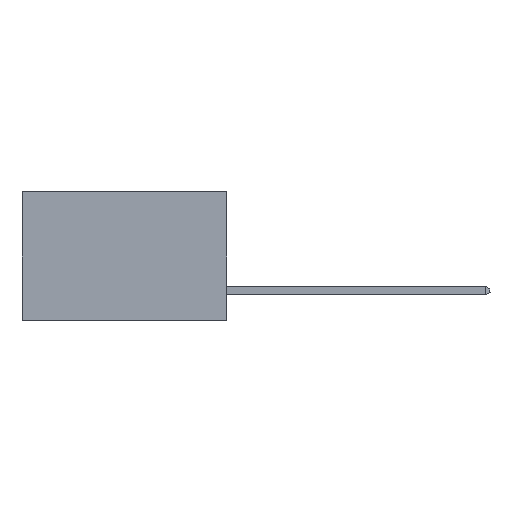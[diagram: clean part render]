
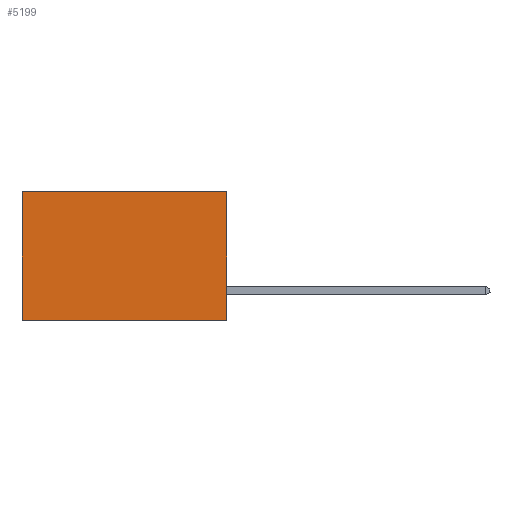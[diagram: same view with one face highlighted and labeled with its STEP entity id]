
A CAD part, left-side view. The second image highlights one B-rep face of the part: STEP entity #5199.
In plain terms, the highlighted planar face has unit normal (-1, 0, 0).
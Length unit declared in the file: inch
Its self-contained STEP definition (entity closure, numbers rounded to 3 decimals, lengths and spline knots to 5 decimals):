
#1485 = DIRECTION ( 'NONE',  ( 0., 0., -1. ) ) ;
#2956 = VECTOR ( 'NONE', #1485, 39.37008 ) ;
#3455 = VECTOR ( 'NONE', #25457, 39.37008 ) ;
#3611 = ORIENTED_EDGE ( 'NONE', *, *, #24521, .F. ) ;
#3801 = ORIENTED_EDGE ( 'NONE', *, *, #17152, .F. ) ;
#4109 = LINE ( 'NONE', #10531, #3455 ) ;
#5102 = VERTEX_POINT ( 'NONE', #23926 ) ;
#5199 = ADVANCED_FACE ( 'NONE', ( #27490 ), #24776, .F. ) ;
#7555 = DIRECTION ( 'NONE',  ( 0., 0., -1. ) ) ;
#8390 = ORIENTED_EDGE ( 'NONE', *, *, #14774, .T. ) ;
#8957 = CARTESIAN_POINT ( 'NONE',  ( 0.277, 0., 0. ) ) ;
#9370 = ORIENTED_EDGE ( 'NONE', *, *, #12000, .T. ) ;
#9481 = VERTEX_POINT ( 'NONE', #24325 ) ;
#9570 = CARTESIAN_POINT ( 'NONE',  ( 0.277, 0., -0.37 ) ) ;
#9664 = VERTEX_POINT ( 'NONE', #16225 ) ;
#9838 = CARTESIAN_POINT ( 'NONE',  ( 0.277, 0., -0.37 ) ) ;
#10531 = CARTESIAN_POINT ( 'NONE',  ( 0.277, 0.59, -0.37 ) ) ;
#10856 = DIRECTION ( 'NONE',  ( 0., 1., 0. ) ) ;
#10966 = LINE ( 'NONE', #8957, #16633 ) ;
#12000 = EDGE_CURVE ( 'NONE', #9481, #5102, #10966, .T. ) ;
#14703 = EDGE_LOOP ( 'NONE', ( #8390, #3611, #3801, #9370 ) ) ;
#14774 = EDGE_CURVE ( 'NONE', #5102, #9664, #4109, .T. ) ;
#16225 = CARTESIAN_POINT ( 'NONE',  ( 0.277, 0.59, -0.37 ) ) ;
#16274 = DIRECTION ( 'NONE',  ( 0., 1., 0. ) ) ;
#16633 = VECTOR ( 'NONE', #10856, 39.37008 ) ;
#17152 = EDGE_CURVE ( 'NONE', #9481, #22321, #18694, .T. ) ;
#17768 = DIRECTION ( 'NONE',  ( 1., 0., 0. ) ) ;
#18694 = LINE ( 'NONE', #24976, #2956 ) ;
#20127 = VECTOR ( 'NONE', #16274, 39.37008 ) ;
#22321 = VERTEX_POINT ( 'NONE', #26163 ) ;
#23899 = AXIS2_PLACEMENT_3D ( 'NONE', #9570, #17768, #7555 ) ;
#23926 = CARTESIAN_POINT ( 'NONE',  ( 0.277, 0.59, 0. ) ) ;
#24325 = CARTESIAN_POINT ( 'NONE',  ( 0.277, 0., 0. ) ) ;
#24521 = EDGE_CURVE ( 'NONE', #22321, #9664, #25761, .T. ) ;
#24776 = PLANE ( 'NONE',  #23899 ) ;
#24976 = CARTESIAN_POINT ( 'NONE',  ( 0.277, 0., -0.37 ) ) ;
#25457 = DIRECTION ( 'NONE',  ( 0., 0., -1. ) ) ;
#25761 = LINE ( 'NONE', #9838, #20127 ) ;
#26163 = CARTESIAN_POINT ( 'NONE',  ( 0.277, 0., -0.37 ) ) ;
#27490 = FACE_OUTER_BOUND ( 'NONE', #14703, .T. ) ;
